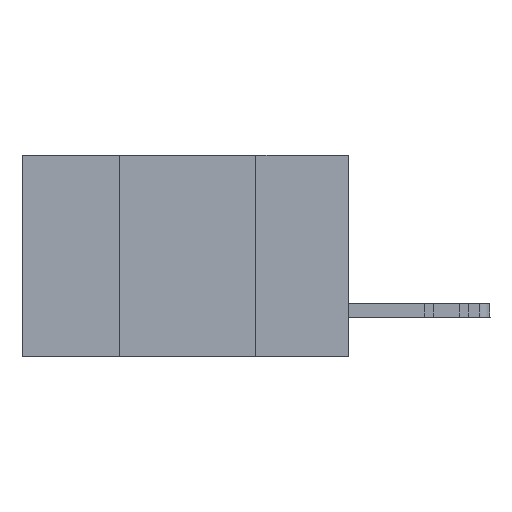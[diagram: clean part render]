
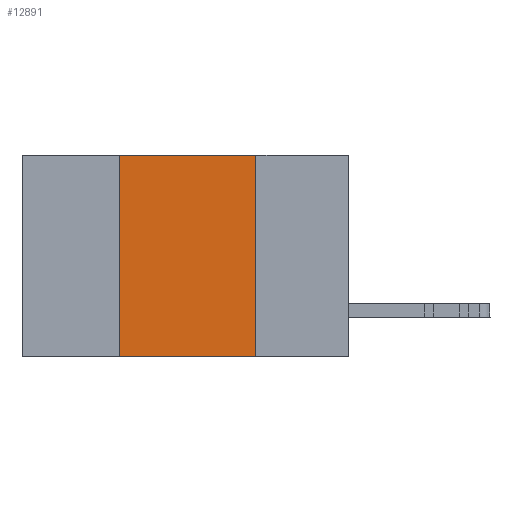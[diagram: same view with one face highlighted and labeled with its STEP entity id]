
A CAD part, left-side view. The second image highlights one B-rep face of the part: STEP entity #12891.
In plain terms, the highlighted planar face has unit normal (-1, 0, 0).
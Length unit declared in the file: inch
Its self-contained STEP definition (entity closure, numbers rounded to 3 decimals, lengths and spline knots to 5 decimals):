
#3 = VECTOR ( 'NONE', #15835, 39.37008 ) ;
#185 = FACE_OUTER_BOUND ( 'NONE', #11369, .T. ) ;
#355 = EDGE_CURVE ( 'NONE', #23587, #18559, #26491, .T. ) ;
#399 = DIRECTION ( 'NONE',  ( 0., 0., 1. ) ) ;
#692 = CARTESIAN_POINT ( 'NONE',  ( 0., 0.17, 0. ) ) ;
#2109 = PLANE ( 'NONE',  #11812 ) ;
#3303 = VECTOR ( 'NONE', #13606, 39.37008 ) ;
#3538 = VERTEX_POINT ( 'NONE', #5159 ) ;
#3872 = DIRECTION ( 'NONE',  ( 1., 0., 0. ) ) ;
#5159 = CARTESIAN_POINT ( 'NONE',  ( 0., 0.17, -0.37 ) ) ;
#5541 = LINE ( 'NONE', #20214, #3 ) ;
#8102 = CARTESIAN_POINT ( 'NONE',  ( 0., 0.6, 0. ) ) ;
#9318 = CARTESIAN_POINT ( 'NONE',  ( 0., 0.6, -0.37 ) ) ;
#9523 = EDGE_CURVE ( 'NONE', #14498, #3538, #23778, .T. ) ;
#9548 = VECTOR ( 'NONE', #399, 39.37008 ) ;
#10439 = CARTESIAN_POINT ( 'NONE',  ( 0., 0.42, -0.37 ) ) ;
#10507 = CARTESIAN_POINT ( 'NONE',  ( 0., 0.42, 0. ) ) ;
#11369 = EDGE_LOOP ( 'NONE', ( #20294, #19351, #13581, #26544 ) ) ;
#11406 = VECTOR ( 'NONE', #24852, 39.37008 ) ;
#11812 = AXIS2_PLACEMENT_3D ( 'NONE', #8102, #3872, #18384 ) ;
#12891 = ADVANCED_FACE ( 'NONE', ( #185 ), #2109, .F. ) ;
#13581 = ORIENTED_EDGE ( 'NONE', *, *, #355, .F. ) ;
#13606 = DIRECTION ( 'NONE',  ( 0., -1., 0. ) ) ;
#14498 = VERTEX_POINT ( 'NONE', #692 ) ;
#15835 = DIRECTION ( 'NONE',  ( 0., -1., 0. ) ) ;
#18384 = DIRECTION ( 'NONE',  ( 0., 0., -1. ) ) ;
#18559 = VERTEX_POINT ( 'NONE', #18953 ) ;
#18953 = CARTESIAN_POINT ( 'NONE',  ( 0., 0.42, 0. ) ) ;
#19206 = EDGE_CURVE ( 'NONE', #23587, #3538, #23122, .T. ) ;
#19351 = ORIENTED_EDGE ( 'NONE', *, *, #26745, .F. ) ;
#20214 = CARTESIAN_POINT ( 'NONE',  ( 0., 0.6, 0. ) ) ;
#20294 = ORIENTED_EDGE ( 'NONE', *, *, #9523, .F. ) ;
#23122 = LINE ( 'NONE', #9318, #3303 ) ;
#23587 = VERTEX_POINT ( 'NONE', #10439 ) ;
#23778 = LINE ( 'NONE', #26939, #11406 ) ;
#24852 = DIRECTION ( 'NONE',  ( 0., 0., -1. ) ) ;
#26491 = LINE ( 'NONE', #10507, #9548 ) ;
#26544 = ORIENTED_EDGE ( 'NONE', *, *, #19206, .T. ) ;
#26745 = EDGE_CURVE ( 'NONE', #18559, #14498, #5541, .T. ) ;
#26939 = CARTESIAN_POINT ( 'NONE',  ( 0., 0.17, 0. ) ) ;
